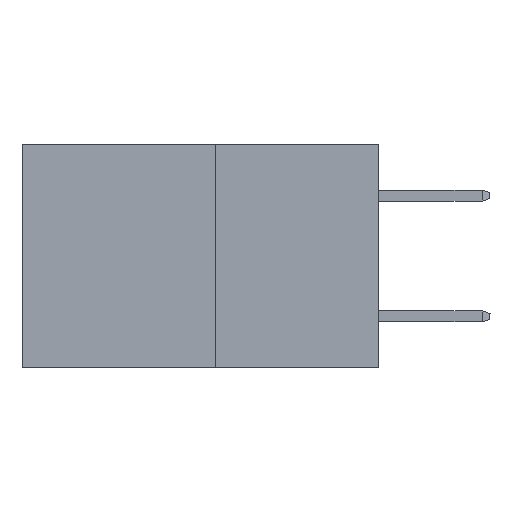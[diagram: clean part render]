
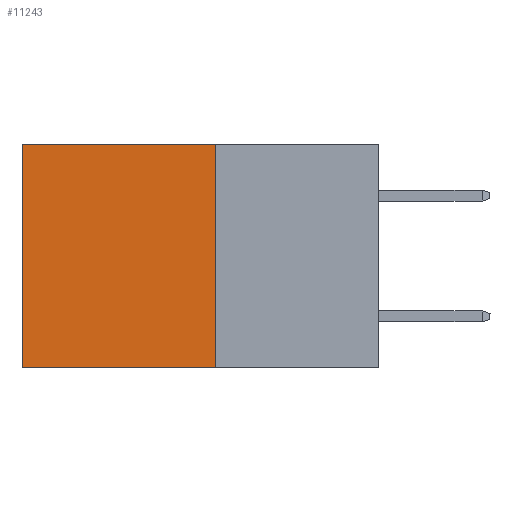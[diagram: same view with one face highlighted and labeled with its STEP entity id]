
A CAD part, left-side view. The second image highlights one B-rep face of the part: STEP entity #11243.
In plain terms, the highlighted planar face has unit normal (-1, 0, 0).
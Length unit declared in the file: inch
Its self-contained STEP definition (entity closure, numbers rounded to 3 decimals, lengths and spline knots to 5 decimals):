
#38 = FACE_OUTER_BOUND ( 'NONE', #5791, .T. ) ;
#102 = LINE ( 'NONE', #5173, #14365 ) ;
#446 = VECTOR ( 'NONE', #6134, 39.37008 ) ;
#618 = CARTESIAN_POINT ( 'NONE',  ( 0.277, 0.27, -0.37 ) ) ;
#1201 = EDGE_CURVE ( 'NONE', #13102, #10476, #5639, .T. ) ;
#1834 = CARTESIAN_POINT ( 'NONE',  ( 0.277, 0.59, -0.37 ) ) ;
#2347 = DIRECTION ( 'NONE',  ( 0., 1., 0. ) ) ;
#2577 = CARTESIAN_POINT ( 'NONE',  ( 0.277, 0.27, 0. ) ) ;
#3232 = ORIENTED_EDGE ( 'NONE', *, *, #12109, .F. ) ;
#5173 = CARTESIAN_POINT ( 'NONE',  ( 0.277, 0.59, -0.37 ) ) ;
#5187 = DIRECTION ( 'NONE',  ( 1., 0., 0. ) ) ;
#5521 = ORIENTED_EDGE ( 'NONE', *, *, #1201, .T. ) ;
#5639 = LINE ( 'NONE', #16104, #8422 ) ;
#5791 = EDGE_LOOP ( 'NONE', ( #10436, #3232, #12460, #5521 ) ) ;
#6134 = DIRECTION ( 'NONE',  ( 0., 1., 0. ) ) ;
#6268 = CARTESIAN_POINT ( 'NONE',  ( 0.277, 0.59, 0. ) ) ;
#6626 = CARTESIAN_POINT ( 'NONE',  ( 0.277, 0.27, -0.37 ) ) ;
#8000 = PLANE ( 'NONE',  #9053 ) ;
#8422 = VECTOR ( 'NONE', #2347, 39.37008 ) ;
#8904 = DIRECTION ( 'NONE',  ( 0., 0., -1. ) ) ;
#9053 = AXIS2_PLACEMENT_3D ( 'NONE', #6626, #5187, #17650 ) ;
#10177 = LINE ( 'NONE', #618, #13405 ) ;
#10436 = ORIENTED_EDGE ( 'NONE', *, *, #15005, .T. ) ;
#10476 = VERTEX_POINT ( 'NONE', #6268 ) ;
#11243 = ADVANCED_FACE ( 'NONE', ( #38 ), #8000, .F. ) ;
#11247 = CARTESIAN_POINT ( 'NONE',  ( 0.277, 0.27, -0.37 ) ) ;
#12041 = VERTEX_POINT ( 'NONE', #1834 ) ;
#12109 = EDGE_CURVE ( 'NONE', #16682, #12041, #14708, .T. ) ;
#12460 = ORIENTED_EDGE ( 'NONE', *, *, #16866, .F. ) ;
#13102 = VERTEX_POINT ( 'NONE', #2577 ) ;
#13405 = VECTOR ( 'NONE', #8904, 39.37008 ) ;
#14365 = VECTOR ( 'NONE', #14805, 39.37008 ) ;
#14369 = CARTESIAN_POINT ( 'NONE',  ( 0.277, 0.27, -0.37 ) ) ;
#14708 = LINE ( 'NONE', #14369, #446 ) ;
#14805 = DIRECTION ( 'NONE',  ( 0., 0., -1. ) ) ;
#15005 = EDGE_CURVE ( 'NONE', #10476, #12041, #102, .T. ) ;
#16104 = CARTESIAN_POINT ( 'NONE',  ( 0.277, 0.27, 0. ) ) ;
#16682 = VERTEX_POINT ( 'NONE', #11247 ) ;
#16866 = EDGE_CURVE ( 'NONE', #13102, #16682, #10177, .T. ) ;
#17650 = DIRECTION ( 'NONE',  ( 0., 0., -1. ) ) ;
